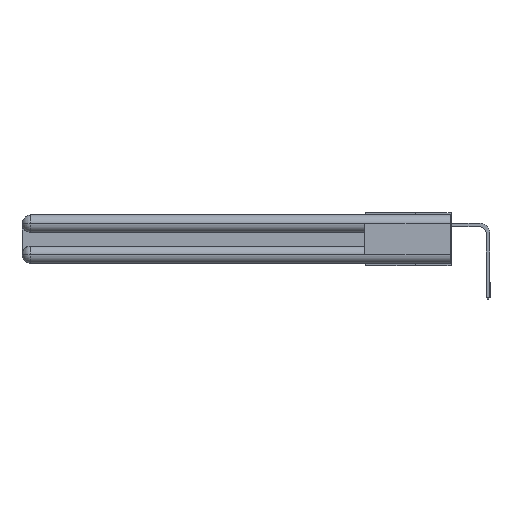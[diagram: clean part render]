
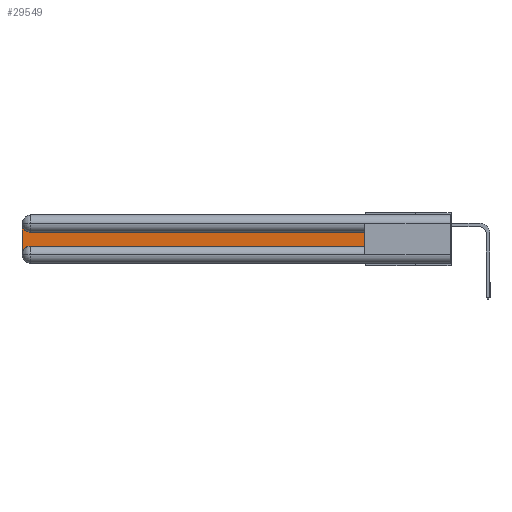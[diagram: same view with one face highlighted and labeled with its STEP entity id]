
A CAD part, left-side view. The second image highlights one B-rep face of the part: STEP entity #29549.
In plain terms, the highlighted planar face has unit normal (-1, 0, 0).
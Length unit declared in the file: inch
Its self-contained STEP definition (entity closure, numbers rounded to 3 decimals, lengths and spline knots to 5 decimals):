
#219 = VECTOR ( 'NONE', #18231, 39.37008 ) ;
#641 = LINE ( 'NONE', #20881, #219 ) ;
#1462 = DIRECTION ( 'NONE',  ( 0., 0., 1. ) ) ;
#4002 = CARTESIAN_POINT ( 'NONE',  ( 0.075, 2.94, -0.0625 ) ) ;
#4273 = VECTOR ( 'NONE', #11824, 39.37008 ) ;
#4321 = VERTEX_POINT ( 'NONE', #18879 ) ;
#5373 = PLANE ( 'NONE',  #7588 ) ;
#5401 = CARTESIAN_POINT ( 'NONE',  ( 0.075, 2.94, -0.2775 ) ) ;
#7073 = CARTESIAN_POINT ( 'NONE',  ( 0.075, 3., -0.2775 ) ) ;
#7507 = LINE ( 'NONE', #19088, #12644 ) ;
#7580 = FACE_OUTER_BOUND ( 'NONE', #28823, .T. ) ;
#7588 = AXIS2_PLACEMENT_3D ( 'NONE', #25590, #20595, #15311 ) ;
#7909 = VERTEX_POINT ( 'NONE', #14424 ) ;
#9235 = VECTOR ( 'NONE', #29212, 39.37008 ) ;
#10680 = AXIS2_PLACEMENT_3D ( 'NONE', #5401, #27922, #13113 ) ;
#11388 = DIRECTION ( 'NONE',  ( 1., 0., 0. ) ) ;
#11711 = VERTEX_POINT ( 'NONE', #24963 ) ;
#11824 = DIRECTION ( 'NONE',  ( 0., 0., -1. ) ) ;
#12271 = EDGE_CURVE ( 'NONE', #4321, #7909, #27852, .T. ) ;
#12644 = VECTOR ( 'NONE', #1462, 39.37008 ) ;
#13022 = EDGE_CURVE ( 'NONE', #14721, #11711, #14817, .T. ) ;
#13113 = DIRECTION ( 'NONE',  ( 0., 0., -1. ) ) ;
#14010 = EDGE_CURVE ( 'NONE', #16549, #4321, #21849, .T. ) ;
#14303 = CARTESIAN_POINT ( 'NONE',  ( 0.075, 0.6, -0.2175 ) ) ;
#14424 = CARTESIAN_POINT ( 'NONE',  ( 0.075, 0.6, -0.2175 ) ) ;
#14721 = VERTEX_POINT ( 'NONE', #18134 ) ;
#14817 = CIRCLE ( 'NONE', #23978, 0.06 ) ;
#15311 = DIRECTION ( 'NONE',  ( 0., 0., -1. ) ) ;
#16549 = VERTEX_POINT ( 'NONE', #7073 ) ;
#17584 = EDGE_CURVE ( 'NONE', #11711, #16549, #18506, .T. ) ;
#18134 = CARTESIAN_POINT ( 'NONE',  ( 0.075, 2.94, -0.1225 ) ) ;
#18231 = DIRECTION ( 'NONE',  ( 0., 1., 0. ) ) ;
#18506 = LINE ( 'NONE', #31917, #4273 ) ;
#18879 = CARTESIAN_POINT ( 'NONE',  ( 0.075, 2.94, -0.2175 ) ) ;
#19088 = CARTESIAN_POINT ( 'NONE',  ( 0.075, 0.6, -0.2175 ) ) ;
#19807 = EDGE_CURVE ( 'NONE', #20985, #14721, #641, .T. ) ;
#20174 = ORIENTED_EDGE ( 'NONE', *, *, #26671, .T. ) ;
#20595 = DIRECTION ( 'NONE',  ( 1., 0., 0. ) ) ;
#20881 = CARTESIAN_POINT ( 'NONE',  ( 0.075, 0.6, -0.1225 ) ) ;
#20985 = VERTEX_POINT ( 'NONE', #26229 ) ;
#21439 = DIRECTION ( 'NONE',  ( 0., 0., -1. ) ) ;
#21849 = CIRCLE ( 'NONE', #10680, 0.06 ) ;
#23768 = ORIENTED_EDGE ( 'NONE', *, *, #13022, .T. ) ;
#23978 = AXIS2_PLACEMENT_3D ( 'NONE', #4002, #11388, #21439 ) ;
#24963 = CARTESIAN_POINT ( 'NONE',  ( 0.075, 3., -0.0625 ) ) ;
#25129 = ORIENTED_EDGE ( 'NONE', *, *, #12271, .T. ) ;
#25590 = CARTESIAN_POINT ( 'NONE',  ( 0.075, 3., -0.1225 ) ) ;
#26229 = CARTESIAN_POINT ( 'NONE',  ( 0.075, 0.6, -0.1225 ) ) ;
#26399 = ORIENTED_EDGE ( 'NONE', *, *, #19807, .T. ) ;
#26671 = EDGE_CURVE ( 'NONE', #7909, #20985, #7507, .T. ) ;
#27852 = LINE ( 'NONE', #14303, #9235 ) ;
#27922 = DIRECTION ( 'NONE',  ( 1., 0., 0. ) ) ;
#28823 = EDGE_LOOP ( 'NONE', ( #26399, #23768, #29335, #30281, #25129, #20174 ) ) ;
#29212 = DIRECTION ( 'NONE',  ( 0., -1., 0. ) ) ;
#29335 = ORIENTED_EDGE ( 'NONE', *, *, #17584, .T. ) ;
#29549 = ADVANCED_FACE ( 'NONE', ( #7580 ), #5373, .F. ) ;
#30281 = ORIENTED_EDGE ( 'NONE', *, *, #14010, .T. ) ;
#31917 = CARTESIAN_POINT ( 'NONE',  ( 0.075, 3., -0.2175 ) ) ;
